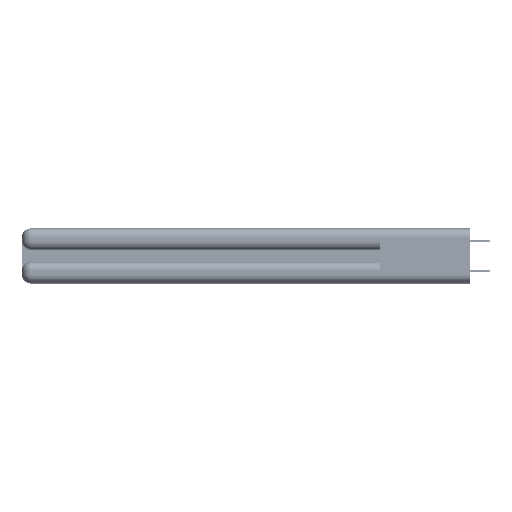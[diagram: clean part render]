
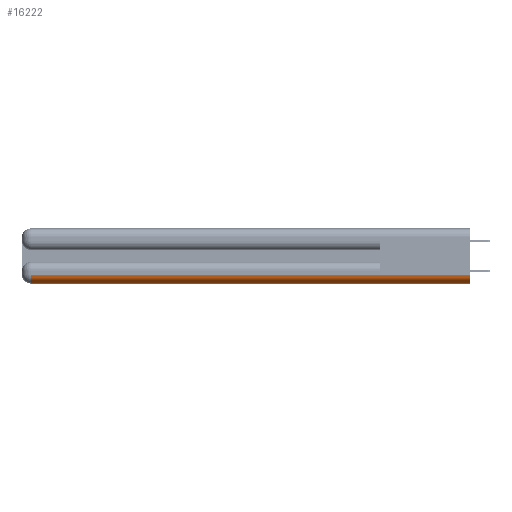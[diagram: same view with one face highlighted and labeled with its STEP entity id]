
A CAD part, left-side view. The second image highlights one B-rep face of the part: STEP entity #16222.
In plain terms, the highlighted cylindrical face has radius 1.524 mm (diameter 3.048 mm), a partial arc.
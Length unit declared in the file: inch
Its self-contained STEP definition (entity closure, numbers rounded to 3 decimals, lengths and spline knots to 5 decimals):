
#1242 = VERTEX_POINT ( 'NONE', #54901 ) ;
#1596 = DIRECTION ( 'NONE',  ( 0., 1., 0. ) ) ;
#1880 = CARTESIAN_POINT ( 'NONE',  ( 0.06, 2.94, 0.06 ) ) ;
#2156 = DIRECTION ( 'NONE',  ( 0., 0., 1. ) ) ;
#4695 = CARTESIAN_POINT ( 'NONE',  ( 0., 2.94, 0.06 ) ) ;
#4961 = CARTESIAN_POINT ( 'NONE',  ( 0.06, 0., 0.06 ) ) ;
#5209 = EDGE_CURVE ( 'NONE', #28785, #1242, #23410, .T. ) ;
#6055 = VECTOR ( 'NONE', #29406, 39.37008 ) ;
#6656 = VERTEX_POINT ( 'NONE', #52722 ) ;
#11738 = CARTESIAN_POINT ( 'NONE',  ( 0., 0., 0.06 ) ) ;
#16222 = ADVANCED_FACE ( 'NONE', ( #26950 ), #44579, .T. ) ;
#17423 = AXIS2_PLACEMENT_3D ( 'NONE', #4961, #22587, #40235 ) ;
#20175 = EDGE_LOOP ( 'NONE', ( #31711, #23303, #54749, #45796 ) ) ;
#22587 = DIRECTION ( 'NONE',  ( 0., 1., 0. ) ) ;
#22951 = AXIS2_PLACEMENT_3D ( 'NONE', #26560, #56884, #26273 ) ;
#23303 = ORIENTED_EDGE ( 'NONE', *, *, #39352, .F. ) ;
#23410 = LINE ( 'NONE', #49453, #46443 ) ;
#23418 = VERTEX_POINT ( 'NONE', #4695 ) ;
#26273 = DIRECTION ( 'NONE',  ( 0., 0., 1. ) ) ;
#26560 = CARTESIAN_POINT ( 'NONE',  ( 0.06, 0., 0.06 ) ) ;
#26950 = FACE_OUTER_BOUND ( 'NONE', #20175, .T. ) ;
#28785 = VERTEX_POINT ( 'NONE', #51152 ) ;
#29406 = DIRECTION ( 'NONE',  ( 0., -1., 0. ) ) ;
#31711 = ORIENTED_EDGE ( 'NONE', *, *, #53527, .F. ) ;
#32888 = LINE ( 'NONE', #11738, #6055 ) ;
#39352 = EDGE_CURVE ( 'NONE', #23418, #6656, #32888, .T. ) ;
#40235 = DIRECTION ( 'NONE',  ( 0., 0., 1. ) ) ;
#42498 = CIRCLE ( 'NONE', #49849, 0.06 ) ;
#44579 = CYLINDRICAL_SURFACE ( 'NONE', #17423, 0.06 ) ;
#45796 = ORIENTED_EDGE ( 'NONE', *, *, #5209, .F. ) ;
#46443 = VECTOR ( 'NONE', #50299, 39.37008 ) ;
#46498 = EDGE_CURVE ( 'NONE', #1242, #23418, #42498, .T. ) ;
#47913 = CIRCLE ( 'NONE', #22951, 0.06 ) ;
#49453 = CARTESIAN_POINT ( 'NONE',  ( 0.06, 3., 0. ) ) ;
#49849 = AXIS2_PLACEMENT_3D ( 'NONE', #1880, #1596, #2156 ) ;
#50299 = DIRECTION ( 'NONE',  ( 0., 1., 0. ) ) ;
#51152 = CARTESIAN_POINT ( 'NONE',  ( 0.06, 0., 0. ) ) ;
#52722 = CARTESIAN_POINT ( 'NONE',  ( 0., 0., 0.06 ) ) ;
#53527 = EDGE_CURVE ( 'NONE', #6656, #28785, #47913, .T. ) ;
#54749 = ORIENTED_EDGE ( 'NONE', *, *, #46498, .F. ) ;
#54901 = CARTESIAN_POINT ( 'NONE',  ( 0.06, 2.94, 0. ) ) ;
#56884 = DIRECTION ( 'NONE',  ( 0., -1., 0. ) ) ;
